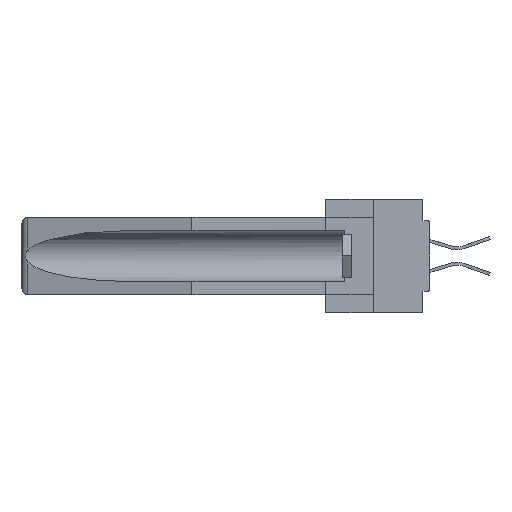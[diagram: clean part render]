
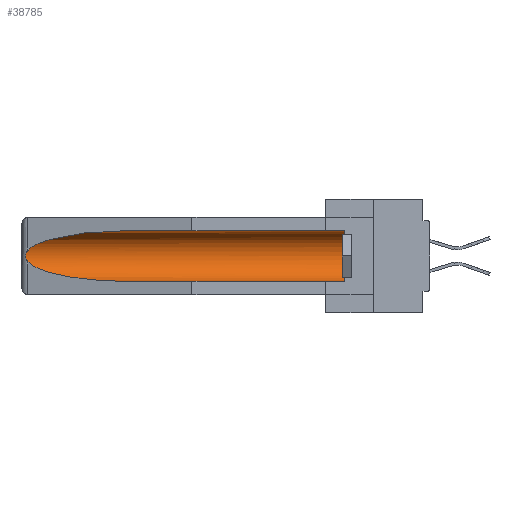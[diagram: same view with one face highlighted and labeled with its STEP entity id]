
A CAD part, left-side view. The second image highlights one B-rep face of the part: STEP entity #38785.
In plain terms, the highlighted cylindrical face has radius 2.857 mm (diameter 5.715 mm), a partial arc.
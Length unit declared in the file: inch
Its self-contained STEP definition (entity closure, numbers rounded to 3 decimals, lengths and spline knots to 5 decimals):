
#206 = EDGE_CURVE ( 'NONE', #9897, #29953, #4163, .T. ) ;
#596 = CARTESIAN_POINT ( 'NONE',  ( 0.26537, 1.52718, -0.19328 ) ) ;
#704 = CARTESIAN_POINT ( 'NONE',  ( 0.26597, 1.5296, -0.19026 ) ) ;
#776 = CARTESIAN_POINT ( 'NONE',  ( 0.155, 1.07973, -0.059 ) ) ;
#929 = CARTESIAN_POINT ( 'NONE',  ( 0.25451, 1.48313, -0.24835 ) ) ;
#1581 = AXIS2_PLACEMENT_3D ( 'NONE', #19768, #37663, #35050 ) ;
#1598 = LINE ( 'NONE', #38055, #12899 ) ;
#2933 = CARTESIAN_POINT ( 'NONE',  ( 0.26537, 1.52718, -0.14972 ) ) ;
#3684 =( BOUNDED_CURVE ( )  B_SPLINE_CURVE ( 3, ( #26815, #17838, #9167, #30264 ),
 .UNSPECIFIED., .F., .T. ) 
 B_SPLINE_CURVE_WITH_KNOTS ( ( 4, 4 ),
 ( 4.71239, 6.08839 ),
 .UNSPECIFIED. ) 
 CURVE ( )  GEOMETRIC_REPRESENTATION_ITEM ( )  RATIONAL_B_SPLINE_CURVE ( ( 1., 0.848, 0.848, 1. ) ) 
 REPRESENTATION_ITEM ( '' )  );
#3726 = VECTOR ( 'NONE', #8107, 39.37008 ) ;
#4163 = CIRCLE ( 'NONE', #1581, 0.1125 ) ;
#5045 = VERTEX_POINT ( 'NONE', #11404 ) ;
#8107 = DIRECTION ( 'NONE',  ( 0., 1., 0. ) ) ;
#9077 = CYLINDRICAL_SURFACE ( 'NONE', #31076, 0.1125 ) ;
#9114 = FACE_OUTER_BOUND ( 'NONE', #23480, .T. ) ;
#9167 = CARTESIAN_POINT ( 'NONE',  ( 0.25451, 1.48313, -0.09465 ) ) ;
#9379 = CARTESIAN_POINT ( 'NONE',  ( 0.26655, 1.53094, -0.18657 ) ) ;
#9513 = CARTESIAN_POINT ( 'NONE',  ( 0.2675, 1.53308, -0.17534 ) ) ;
#9897 = VERTEX_POINT ( 'NONE', #22570 ) ;
#11404 = CARTESIAN_POINT ( 'NONE',  ( 0.155, 1.07973, -0.284 ) ) ;
#12785 = CARTESIAN_POINT ( 'NONE',  ( 0.2675, 1.53308, -0.16763 ) ) ;
#12899 = VECTOR ( 'NONE', #20160, 39.37008 ) ;
#12972 = EDGE_CURVE ( 'NONE', #9897, #5045, #1598, .T. ) ;
#13197 = DIRECTION ( 'NONE',  ( 0., 0., 1. ) ) ;
#14251 =( BOUNDED_CURVE ( )  B_SPLINE_CURVE ( 3, ( #21312, #929, #36836, #22111 ),
 .UNSPECIFIED., .F., .T. ) 
 B_SPLINE_CURVE_WITH_KNOTS ( ( 4, 4 ),
 ( 0.1948, 1.5708 ),
 .UNSPECIFIED. ) 
 CURVE ( )  GEOMETRIC_REPRESENTATION_ITEM ( )  RATIONAL_B_SPLINE_CURVE ( ( 1., 0.848, 0.848, 1. ) ) 
 REPRESENTATION_ITEM ( '' )  );
#15929 = LINE ( 'NONE', #38753, #3726 ) ;
#16850 = ORIENTED_EDGE ( 'NONE', *, *, #24060, .T. ) ;
#17783 = CARTESIAN_POINT ( 'NONE',  ( 0.26537, 1.52718, -0.19328 ) ) ;
#17838 = CARTESIAN_POINT ( 'NONE',  ( 0.21114, 1.30732, -0.059 ) ) ;
#18452 = CARTESIAN_POINT ( 'NONE',  ( 0.26654, 1.53092, -0.15636 ) ) ;
#19110 = DIRECTION ( 'NONE',  ( 0., 1., 0. ) ) ;
#19768 = CARTESIAN_POINT ( 'NONE',  ( 0.155, 0.126, -0.1715 ) ) ;
#20043 = EDGE_CURVE ( 'NONE', #22988, #5045, #14251, .T. ) ;
#20160 = DIRECTION ( 'NONE',  ( 0., 1., 0. ) ) ;
#21312 = CARTESIAN_POINT ( 'NONE',  ( 0.26537, 1.52718, -0.19328 ) ) ;
#22111 = CARTESIAN_POINT ( 'NONE',  ( 0.155, 1.07973, -0.284 ) ) ;
#22332 = VERTEX_POINT ( 'NONE', #776 ) ;
#22570 = CARTESIAN_POINT ( 'NONE',  ( 0.155, 0.126, -0.284 ) ) ;
#22988 = VERTEX_POINT ( 'NONE', #17783 ) ;
#22993 = ORIENTED_EDGE ( 'NONE', *, *, #206, .T. ) ;
#23480 = EDGE_LOOP ( 'NONE', ( #36543, #26718, #38159, #35954, #22993, #16850 ) ) ;
#24060 = EDGE_CURVE ( 'NONE', #29953, #22332, #15929, .T. ) ;
#24177 = EDGE_CURVE ( 'NONE', #22332, #27668, #3684, .T. ) ;
#25562 = CARTESIAN_POINT ( 'NONE',  ( 0.155, 0.126, -0.059 ) ) ;
#26718 = ORIENTED_EDGE ( 'NONE', *, *, #27834, .T. ) ;
#26815 = CARTESIAN_POINT ( 'NONE',  ( 0.155, 1.07973, -0.059 ) ) ;
#27431 = CARTESIAN_POINT ( 'NONE',  ( 0.26597, 1.52961, -0.15275 ) ) ;
#27668 = VERTEX_POINT ( 'NONE', #2933 ) ;
#27834 = EDGE_CURVE ( 'NONE', #27668, #22988, #36935, .T. ) ;
#29953 = VERTEX_POINT ( 'NONE', #25562 ) ;
#30264 = CARTESIAN_POINT ( 'NONE',  ( 0.26537, 1.52718, -0.14972 ) ) ;
#31076 = AXIS2_PLACEMENT_3D ( 'NONE', #37140, #19110, #13197 ) ;
#33466 = CARTESIAN_POINT ( 'NONE',  ( 0.26537, 1.52718, -0.14972 ) ) ;
#33861 = CARTESIAN_POINT ( 'NONE',  ( 0.2673, 1.53269, -0.17917 ) ) ;
#35050 = DIRECTION ( 'NONE',  ( 0., 0., 1. ) ) ;
#35954 = ORIENTED_EDGE ( 'NONE', *, *, #12972, .F. ) ;
#36543 = ORIENTED_EDGE ( 'NONE', *, *, #24177, .T. ) ;
#36593 = CARTESIAN_POINT ( 'NONE',  ( 0.2673, 1.5327, -0.16383 ) ) ;
#36836 = CARTESIAN_POINT ( 'NONE',  ( 0.21114, 1.30732, -0.284 ) ) ;
#36935 = B_SPLINE_CURVE_WITH_KNOTS ( 'NONE', 3,
 ( #33466, #27431, #18452, #36593, #12785, #9513, #33861, #9379, #704, #596 ),
 .UNSPECIFIED., .F., .F.,
 ( 4, 2, 2, 2, 4 ),
 ( 0., 0.00029, 0.00058, 0.00087, 0.00117 ),
 .UNSPECIFIED. ) ;
#37140 = CARTESIAN_POINT ( 'NONE',  ( 0.155, -0.30754, -0.1715 ) ) ;
#37663 = DIRECTION ( 'NONE',  ( 0., -1., 0. ) ) ;
#38055 = CARTESIAN_POINT ( 'NONE',  ( 0.155, -0.30754, -0.284 ) ) ;
#38159 = ORIENTED_EDGE ( 'NONE', *, *, #20043, .T. ) ;
#38753 = CARTESIAN_POINT ( 'NONE',  ( 0.155, -0.30754, -0.059 ) ) ;
#38785 = ADVANCED_FACE ( 'NONE', ( #9114 ), #9077, .F. ) ;
